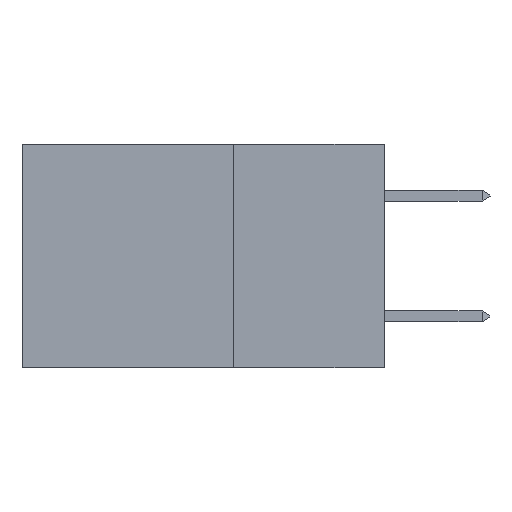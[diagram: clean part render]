
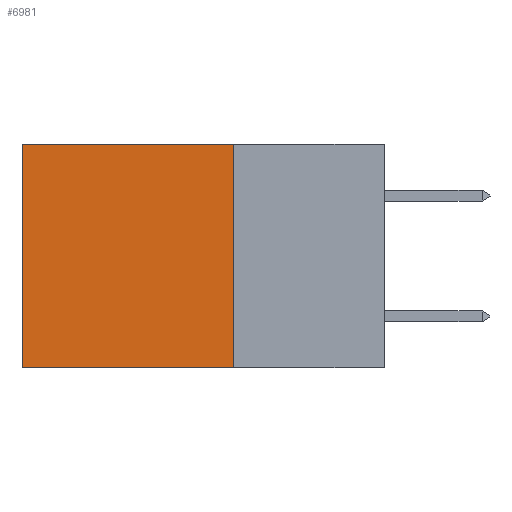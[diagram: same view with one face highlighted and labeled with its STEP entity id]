
A CAD part, left-side view. The second image highlights one B-rep face of the part: STEP entity #6981.
In plain terms, the highlighted planar face has unit normal (-1, 0, 0).
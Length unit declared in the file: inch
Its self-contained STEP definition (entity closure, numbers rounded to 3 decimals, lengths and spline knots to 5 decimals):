
#504 = EDGE_CURVE ( 'NONE', #7113, #1424, #5985, .T. ) ;
#539 = DIRECTION ( 'NONE',  ( 0., 1., 0. ) ) ;
#1317 = VECTOR ( 'NONE', #539, 39.37008 ) ;
#1424 = VERTEX_POINT ( 'NONE', #2907 ) ;
#1448 = CARTESIAN_POINT ( 'NONE',  ( 0.2875, 0.25, 0. ) ) ;
#1503 = DIRECTION ( 'NONE',  ( 0., 0., -1. ) ) ;
#2373 = FACE_OUTER_BOUND ( 'NONE', #5776, .T. ) ;
#2486 = EDGE_CURVE ( 'NONE', #1424, #3892, #5084, .T. ) ;
#2641 = ORIENTED_EDGE ( 'NONE', *, *, #5259, .F. ) ;
#2907 = CARTESIAN_POINT ( 'NONE',  ( 0.2875, 0.6, 0. ) ) ;
#3238 = CARTESIAN_POINT ( 'NONE',  ( 0.2875, 0.25, 0. ) ) ;
#3499 = CARTESIAN_POINT ( 'NONE',  ( 0.2875, 0.25, 0. ) ) ;
#3784 = ORIENTED_EDGE ( 'NONE', *, *, #6724, .F. ) ;
#3892 = VERTEX_POINT ( 'NONE', #10030 ) ;
#4011 = LINE ( 'NONE', #3238, #7318 ) ;
#4071 = DIRECTION ( 'NONE',  ( 0., 1., 0. ) ) ;
#4129 = VERTEX_POINT ( 'NONE', #5078 ) ;
#4600 = ORIENTED_EDGE ( 'NONE', *, *, #2486, .T. ) ;
#4957 = CARTESIAN_POINT ( 'NONE',  ( 0.2875, 0.25, 0. ) ) ;
#5078 = CARTESIAN_POINT ( 'NONE',  ( 0.2875, 0.25, -0.37 ) ) ;
#5084 = LINE ( 'NONE', #5134, #6013 ) ;
#5134 = CARTESIAN_POINT ( 'NONE',  ( 0.2875, 0.6, 0. ) ) ;
#5259 = EDGE_CURVE ( 'NONE', #4129, #3892, #5751, .T. ) ;
#5459 = ORIENTED_EDGE ( 'NONE', *, *, #504, .T. ) ;
#5474 = PLANE ( 'NONE',  #5581 ) ;
#5581 = AXIS2_PLACEMENT_3D ( 'NONE', #1448, #6947, #1503 ) ;
#5751 = LINE ( 'NONE', #7227, #6642 ) ;
#5776 = EDGE_LOOP ( 'NONE', ( #4600, #2641, #3784, #5459 ) ) ;
#5985 = LINE ( 'NONE', #3499, #1317 ) ;
#6013 = VECTOR ( 'NONE', #7535, 39.37008 ) ;
#6642 = VECTOR ( 'NONE', #4071, 39.37008 ) ;
#6724 = EDGE_CURVE ( 'NONE', #7113, #4129, #4011, .T. ) ;
#6947 = DIRECTION ( 'NONE',  ( 1., 0., 0. ) ) ;
#6981 = ADVANCED_FACE ( 'NONE', ( #2373 ), #5474, .F. ) ;
#7113 = VERTEX_POINT ( 'NONE', #4957 ) ;
#7212 = DIRECTION ( 'NONE',  ( 0., 0., -1. ) ) ;
#7227 = CARTESIAN_POINT ( 'NONE',  ( 0.2875, 0.25, -0.37 ) ) ;
#7318 = VECTOR ( 'NONE', #7212, 39.37008 ) ;
#7535 = DIRECTION ( 'NONE',  ( 0., 0., -1. ) ) ;
#10030 = CARTESIAN_POINT ( 'NONE',  ( 0.2875, 0.6, -0.37 ) ) ;
